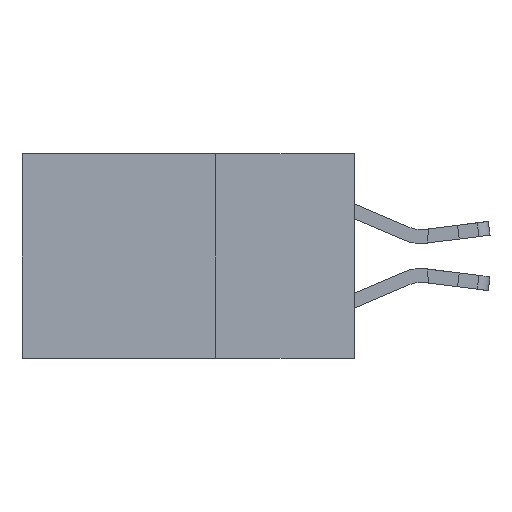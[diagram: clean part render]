
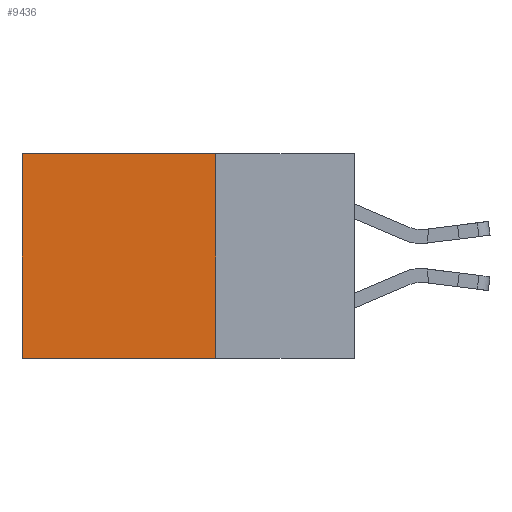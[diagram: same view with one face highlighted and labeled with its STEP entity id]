
A CAD part, left-side view. The second image highlights one B-rep face of the part: STEP entity #9436.
In plain terms, the highlighted planar face has unit normal (-1, 0, 0).
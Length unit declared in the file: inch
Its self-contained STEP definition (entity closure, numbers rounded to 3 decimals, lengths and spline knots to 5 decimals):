
#6 = EDGE_CURVE ( 'NONE', #6525, #8353, #5694, .T. ) ;
#344 = LINE ( 'NONE', #5487, #4235 ) ;
#913 = CARTESIAN_POINT ( 'NONE',  ( 0.2615, 0.6, -0.37 ) ) ;
#1163 = DIRECTION ( 'NONE',  ( 0., 0., -1. ) ) ;
#1246 = EDGE_CURVE ( 'NONE', #8353, #10018, #344, .T. ) ;
#2168 = VECTOR ( 'NONE', #6431, 39.37008 ) ;
#2459 = CARTESIAN_POINT ( 'NONE',  ( 0.2615, 0.6, 0. ) ) ;
#2930 = AXIS2_PLACEMENT_3D ( 'NONE', #8914, #8079, #1163 ) ;
#3697 = DIRECTION ( 'NONE',  ( 0., 0., -1. ) ) ;
#3972 = CARTESIAN_POINT ( 'NONE',  ( 0.2615, 0.25, -0.37 ) ) ;
#4235 = VECTOR ( 'NONE', #3697, 39.37008 ) ;
#4910 = ORIENTED_EDGE ( 'NONE', *, *, #6670, .F. ) ;
#5097 = LINE ( 'NONE', #5264, #6442 ) ;
#5264 = CARTESIAN_POINT ( 'NONE',  ( 0.2615, 0.25, -0.37 ) ) ;
#5328 = CARTESIAN_POINT ( 'NONE',  ( 0.2615, 0.25, 0. ) ) ;
#5487 = CARTESIAN_POINT ( 'NONE',  ( 0.2615, 0.6, -0.37 ) ) ;
#5643 = CARTESIAN_POINT ( 'NONE',  ( 0.2615, 0.25, 0. ) ) ;
#5694 = LINE ( 'NONE', #5643, #10088 ) ;
#5750 = DIRECTION ( 'NONE',  ( 0., 1., 0. ) ) ;
#6431 = DIRECTION ( 'NONE',  ( 0., 0., -1. ) ) ;
#6442 = VECTOR ( 'NONE', #10184, 39.37008 ) ;
#6525 = VERTEX_POINT ( 'NONE', #5328 ) ;
#6670 = EDGE_CURVE ( 'NONE', #6525, #6835, #8927, .T. ) ;
#6835 = VERTEX_POINT ( 'NONE', #3972 ) ;
#6887 = ORIENTED_EDGE ( 'NONE', *, *, #6, .T. ) ;
#6921 = EDGE_CURVE ( 'NONE', #6835, #10018, #5097, .T. ) ;
#6995 = EDGE_LOOP ( 'NONE', ( #10705, #9070, #4910, #6887 ) ) ;
#8079 = DIRECTION ( 'NONE',  ( 1., 0., 0. ) ) ;
#8353 = VERTEX_POINT ( 'NONE', #2459 ) ;
#8914 = CARTESIAN_POINT ( 'NONE',  ( 0.2615, 0.25, -0.37 ) ) ;
#8927 = LINE ( 'NONE', #10684, #2168 ) ;
#9070 = ORIENTED_EDGE ( 'NONE', *, *, #6921, .F. ) ;
#9436 = ADVANCED_FACE ( 'NONE', ( #9848 ), #10504, .F. ) ;
#9848 = FACE_OUTER_BOUND ( 'NONE', #6995, .T. ) ;
#10018 = VERTEX_POINT ( 'NONE', #913 ) ;
#10088 = VECTOR ( 'NONE', #5750, 39.37008 ) ;
#10184 = DIRECTION ( 'NONE',  ( 0., 1., 0. ) ) ;
#10504 = PLANE ( 'NONE',  #2930 ) ;
#10684 = CARTESIAN_POINT ( 'NONE',  ( 0.2615, 0.25, -0.37 ) ) ;
#10705 = ORIENTED_EDGE ( 'NONE', *, *, #1246, .T. ) ;
